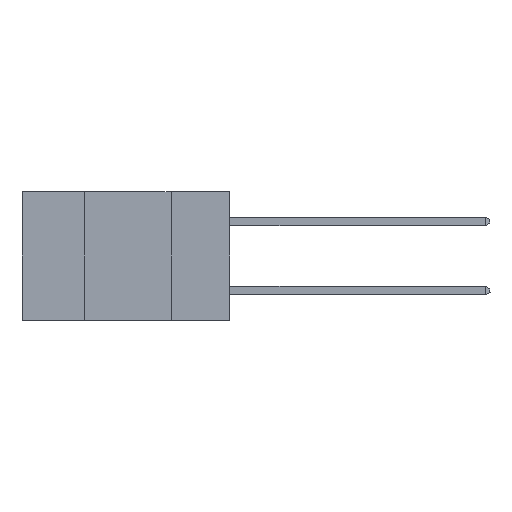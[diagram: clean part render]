
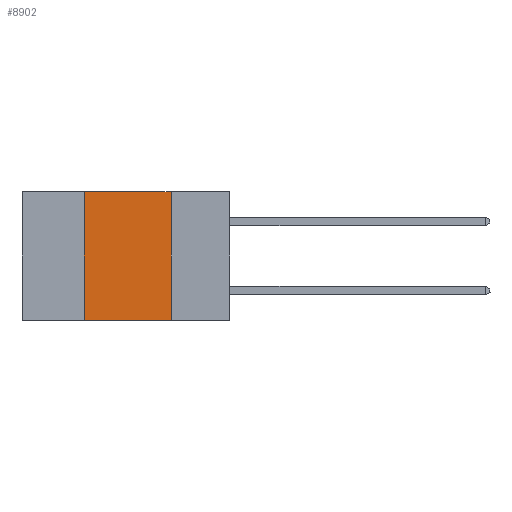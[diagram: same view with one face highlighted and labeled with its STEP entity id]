
A CAD part, left-side view. The second image highlights one B-rep face of the part: STEP entity #8902.
In plain terms, the highlighted planar face has unit normal (-1, 0, 0).
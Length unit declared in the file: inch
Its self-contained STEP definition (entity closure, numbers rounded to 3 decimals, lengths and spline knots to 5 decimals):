
#653 = ORIENTED_EDGE ( 'NONE', *, *, #19940, .F. ) ;
#2035 = DIRECTION ( 'NONE',  ( 0., -1., 0. ) ) ;
#2405 = EDGE_CURVE ( 'NONE', #2818, #9409, #7487, .T. ) ;
#2818 = VERTEX_POINT ( 'NONE', #16914 ) ;
#3206 = EDGE_CURVE ( 'NONE', #9409, #12894, #22043, .T. ) ;
#4718 = CARTESIAN_POINT ( 'NONE',  ( 0., 0.17, 0. ) ) ;
#4885 = DIRECTION ( 'NONE',  ( 0., -1., 0. ) ) ;
#6361 = AXIS2_PLACEMENT_3D ( 'NONE', #20182, #21927, #24033 ) ;
#7487 = LINE ( 'NONE', #13534, #17593 ) ;
#7621 = DIRECTION ( 'NONE',  ( 0., 0., 1. ) ) ;
#8902 = ADVANCED_FACE ( 'NONE', ( #15431 ), #10792, .F. ) ;
#8956 = EDGE_LOOP ( 'NONE', ( #653, #15377, #18744, #9856 ) ) ;
#9409 = VERTEX_POINT ( 'NONE', #10518 ) ;
#9856 = ORIENTED_EDGE ( 'NONE', *, *, #21585, .T. ) ;
#10137 = LINE ( 'NONE', #23190, #21428 ) ;
#10518 = CARTESIAN_POINT ( 'NONE',  ( 0., 0.42, 0. ) ) ;
#10792 = PLANE ( 'NONE',  #6361 ) ;
#12894 = VERTEX_POINT ( 'NONE', #4718 ) ;
#12971 = VECTOR ( 'NONE', #23400, 39.37008 ) ;
#13534 = CARTESIAN_POINT ( 'NONE',  ( 0., 0.42, 0. ) ) ;
#14016 = VECTOR ( 'NONE', #4885, 39.37008 ) ;
#15207 = VERTEX_POINT ( 'NONE', #21221 ) ;
#15377 = ORIENTED_EDGE ( 'NONE', *, *, #3206, .F. ) ;
#15431 = FACE_OUTER_BOUND ( 'NONE', #8956, .T. ) ;
#16914 = CARTESIAN_POINT ( 'NONE',  ( 0., 0.42, -0.37 ) ) ;
#17593 = VECTOR ( 'NONE', #7621, 39.37008 ) ;
#18744 = ORIENTED_EDGE ( 'NONE', *, *, #2405, .F. ) ;
#19560 = CARTESIAN_POINT ( 'NONE',  ( 0., 0.17, 0. ) ) ;
#19904 = CARTESIAN_POINT ( 'NONE',  ( 0., 0.6, 0. ) ) ;
#19940 = EDGE_CURVE ( 'NONE', #12894, #15207, #20089, .T. ) ;
#20089 = LINE ( 'NONE', #19560, #12971 ) ;
#20182 = CARTESIAN_POINT ( 'NONE',  ( 0., 0.6, 0. ) ) ;
#21221 = CARTESIAN_POINT ( 'NONE',  ( 0., 0.17, -0.37 ) ) ;
#21428 = VECTOR ( 'NONE', #2035, 39.37008 ) ;
#21585 = EDGE_CURVE ( 'NONE', #2818, #15207, #10137, .T. ) ;
#21927 = DIRECTION ( 'NONE',  ( 1., 0., 0. ) ) ;
#22043 = LINE ( 'NONE', #19904, #14016 ) ;
#23190 = CARTESIAN_POINT ( 'NONE',  ( 0., 0.6, -0.37 ) ) ;
#23400 = DIRECTION ( 'NONE',  ( 0., 0., -1. ) ) ;
#24033 = DIRECTION ( 'NONE',  ( 0., 0., -1. ) ) ;
